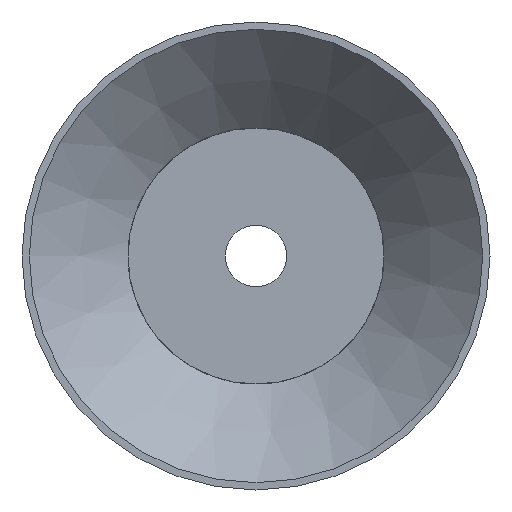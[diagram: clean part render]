
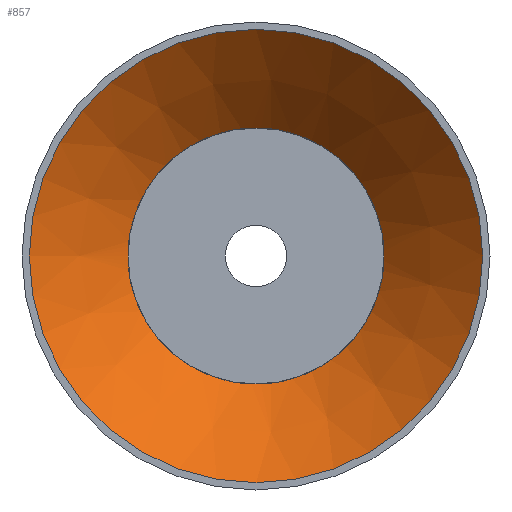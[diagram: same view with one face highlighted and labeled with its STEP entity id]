
A CAD part, front view. The second image highlights one B-rep face of the part: STEP entity #857.
In plain terms, the highlighted conical face has half-angle 44.198 degrees and reference radius 30.725 mm.
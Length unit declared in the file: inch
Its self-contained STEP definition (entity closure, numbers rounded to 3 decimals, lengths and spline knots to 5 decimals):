
#120=(
BOUNDED_CURVE()
B_SPLINE_CURVE(2,(#1166,#1167,#1168),.UNSPECIFIED.,.F.,.F.)
B_SPLINE_CURVE_WITH_KNOTS((3,3),(0.,0.02349),.UNSPECIFIED.)
CURVE()
GEOMETRIC_REPRESENTATION_ITEM()
RATIONAL_B_SPLINE_CURVE((1.,1.,1.))
REPRESENTATION_ITEM('')
);
#121=(
BOUNDED_CURVE()
B_SPLINE_CURVE(2,(#1170,#1171,#1172),.UNSPECIFIED.,.F.,.F.)
B_SPLINE_CURVE_WITH_KNOTS((3,3),(0.83056,0.85405),
 .UNSPECIFIED.)
CURVE()
GEOMETRIC_REPRESENTATION_ITEM()
RATIONAL_B_SPLINE_CURVE((1.,1.,1.))
REPRESENTATION_ITEM('')
);
#122=(
BOUNDED_CURVE()
B_SPLINE_CURVE(2,(#1175,#1176,#1177),.UNSPECIFIED.,.F.,.F.)
B_SPLINE_CURVE_WITH_KNOTS((3,3),(0.,0.02349),.UNSPECIFIED.)
CURVE()
GEOMETRIC_REPRESENTATION_ITEM()
RATIONAL_B_SPLINE_CURVE((1.,1.,1.))
REPRESENTATION_ITEM('')
);
#123=(
BOUNDED_CURVE()
B_SPLINE_CURVE(2,(#1179,#1180,#1181),.UNSPECIFIED.,.F.,.F.)
B_SPLINE_CURVE_WITH_KNOTS((3,3),(0.83035,0.85384),
 .UNSPECIFIED.)
CURVE()
GEOMETRIC_REPRESENTATION_ITEM()
RATIONAL_B_SPLINE_CURVE((1.,1.,1.))
REPRESENTATION_ITEM('')
);
#124=(
BOUNDED_CURVE()
B_SPLINE_CURVE(2,(#1185,#1186,#1187),.UNSPECIFIED.,.F.,.F.)
B_SPLINE_CURVE_WITH_KNOTS((3,3),(0.,0.02349),.UNSPECIFIED.)
CURVE()
GEOMETRIC_REPRESENTATION_ITEM()
RATIONAL_B_SPLINE_CURVE((1.,1.,1.))
REPRESENTATION_ITEM('')
);
#125=(
BOUNDED_CURVE()
B_SPLINE_CURVE(2,(#1191,#1192,#1193),.UNSPECIFIED.,.F.,.F.)
B_SPLINE_CURVE_WITH_KNOTS((3,3),(0.83055,0.85403),
 .UNSPECIFIED.)
CURVE()
GEOMETRIC_REPRESENTATION_ITEM()
RATIONAL_B_SPLINE_CURVE((1.,1.,1.))
REPRESENTATION_ITEM('')
);
#126=(
BOUNDED_CURVE()
B_SPLINE_CURVE(2,(#1196,#1197,#1198),.UNSPECIFIED.,.F.,.F.)
B_SPLINE_CURVE_WITH_KNOTS((3,3),(0.,0.02349),.UNSPECIFIED.)
CURVE()
GEOMETRIC_REPRESENTATION_ITEM()
RATIONAL_B_SPLINE_CURVE((1.,1.,1.))
REPRESENTATION_ITEM('')
);
#127=(
BOUNDED_CURVE()
B_SPLINE_CURVE(2,(#1200,#1201,#1202),.UNSPECIFIED.,.F.,.F.)
B_SPLINE_CURVE_WITH_KNOTS((3,3),(0.83061,0.8541),
 .UNSPECIFIED.)
CURVE()
GEOMETRIC_REPRESENTATION_ITEM()
RATIONAL_B_SPLINE_CURVE((1.,1.,1.))
REPRESENTATION_ITEM('')
);
#132=FACE_OUTER_BOUND('',#172,.T.);
#172=EDGE_LOOP('',(#567,#568,#569,#570,#571,#572,#573,#574,#575,#576,#577,
#578,#579,#580,#581,#582,#583,#584,#585,#586,#587));
#212=CIRCLE('',#910,0.86928);
#214=CIRCLE('',#913,0.86928);
#215=CIRCLE('',#915,0.86928);
#217=CIRCLE('',#918,1.55);
#218=CIRCLE('',#919,0.875);
#219=CIRCLE('',#920,0.875);
#220=CIRCLE('',#921,0.875);
#221=CIRCLE('',#922,0.86928);
#222=CIRCLE('',#923,0.875);
#223=CIRCLE('',#924,0.875);
#224=CIRCLE('',#925,1.55);
#253=LINE('',#1163,#284);
#284=VECTOR('',#1001,1.20964);
#310=VERTEX_POINT('',#1133);
#312=VERTEX_POINT('',#1137);
#314=VERTEX_POINT('',#1142);
#316=VERTEX_POINT('',#1146);
#317=VERTEX_POINT('',#1150);
#319=VERTEX_POINT('',#1153);
#321=VERTEX_POINT('',#1159);
#322=VERTEX_POINT('',#1160);
#323=VERTEX_POINT('',#1162);
#324=VERTEX_POINT('',#1164);
#325=VERTEX_POINT('',#1169);
#326=VERTEX_POINT('',#1173);
#327=VERTEX_POINT('',#1178);
#328=VERTEX_POINT('',#1182);
#329=VERTEX_POINT('',#1184);
#330=VERTEX_POINT('',#1188);
#331=VERTEX_POINT('',#1190);
#332=VERTEX_POINT('',#1194);
#333=VERTEX_POINT('',#1199);
#412=EDGE_CURVE('',#312,#310,#212,.T.);
#416=EDGE_CURVE('',#316,#314,#214,.T.);
#418=EDGE_CURVE('',#317,#319,#215,.T.);
#421=EDGE_CURVE('',#321,#322,#217,.T.);
#422=EDGE_CURVE('',#322,#323,#253,.T.);
#423=EDGE_CURVE('',#324,#323,#218,.T.);
#424=EDGE_CURVE('',#310,#324,#120,.T.);
#425=EDGE_CURVE('',#325,#312,#121,.T.);
#426=EDGE_CURVE('',#326,#325,#219,.T.);
#427=EDGE_CURVE('',#319,#326,#122,.T.);
#428=EDGE_CURVE('',#327,#317,#123,.T.);
#429=EDGE_CURVE('',#328,#327,#220,.T.);
#430=EDGE_CURVE('',#329,#328,#124,.T.);
#431=EDGE_CURVE('',#330,#329,#221,.T.);
#432=EDGE_CURVE('',#331,#330,#125,.T.);
#433=EDGE_CURVE('',#332,#331,#222,.T.);
#434=EDGE_CURVE('',#314,#332,#126,.T.);
#435=EDGE_CURVE('',#333,#316,#127,.T.);
#436=EDGE_CURVE('',#323,#333,#223,.T.);
#437=EDGE_CURVE('',#322,#321,#224,.T.);
#567=ORIENTED_EDGE('',*,*,#421,.T.);
#568=ORIENTED_EDGE('',*,*,#422,.T.);
#569=ORIENTED_EDGE('',*,*,#423,.F.);
#570=ORIENTED_EDGE('',*,*,#424,.F.);
#571=ORIENTED_EDGE('',*,*,#412,.F.);
#572=ORIENTED_EDGE('',*,*,#425,.F.);
#573=ORIENTED_EDGE('',*,*,#426,.F.);
#574=ORIENTED_EDGE('',*,*,#427,.F.);
#575=ORIENTED_EDGE('',*,*,#418,.F.);
#576=ORIENTED_EDGE('',*,*,#428,.F.);
#577=ORIENTED_EDGE('',*,*,#429,.F.);
#578=ORIENTED_EDGE('',*,*,#430,.F.);
#579=ORIENTED_EDGE('',*,*,#431,.F.);
#580=ORIENTED_EDGE('',*,*,#432,.F.);
#581=ORIENTED_EDGE('',*,*,#433,.F.);
#582=ORIENTED_EDGE('',*,*,#434,.F.);
#583=ORIENTED_EDGE('',*,*,#416,.F.);
#584=ORIENTED_EDGE('',*,*,#435,.F.);
#585=ORIENTED_EDGE('',*,*,#436,.F.);
#586=ORIENTED_EDGE('',*,*,#422,.F.);
#587=ORIENTED_EDGE('',*,*,#437,.T.);
#850=CONICAL_SURFACE('',#917,1.20964,0.771);
#857=ADVANCED_FACE('',(#132),#850,.F.);
#910=AXIS2_PLACEMENT_3D('',#1139,#979,#980);
#913=AXIS2_PLACEMENT_3D('',#1148,#987,#988);
#915=AXIS2_PLACEMENT_3D('',#1154,#992,#993);
#917=AXIS2_PLACEMENT_3D('',#1158,#997,#998);
#918=AXIS2_PLACEMENT_3D('',#1161,#999,#1000);
#919=AXIS2_PLACEMENT_3D('',#1165,#1002,#1003);
#920=AXIS2_PLACEMENT_3D('',#1174,#1004,#1005);
#921=AXIS2_PLACEMENT_3D('',#1183,#1006,#1007);
#922=AXIS2_PLACEMENT_3D('',#1189,#1008,#1009);
#923=AXIS2_PLACEMENT_3D('',#1195,#1010,#1011);
#924=AXIS2_PLACEMENT_3D('',#1203,#1012,#1013);
#925=AXIS2_PLACEMENT_3D('',#1204,#1014,#1015);
#979=DIRECTION('center_axis',(0.,-1.,0.));
#980=DIRECTION('ref_axis',(1.,0.,0.));
#987=DIRECTION('center_axis',(0.,-1.,0.));
#988=DIRECTION('ref_axis',(1.,0.,0.));
#992=DIRECTION('center_axis',(0.,-1.,0.));
#993=DIRECTION('ref_axis',(1.,0.,0.));
#997=DIRECTION('center_axis',(0.,-1.,0.));
#998=DIRECTION('ref_axis',(1.,0.,0.));
#999=DIRECTION('center_axis',(0.,-1.,0.));
#1000=DIRECTION('ref_axis',(1.,0.,0.));
#1001=DIRECTION('',(0.697,0.717,0.));
#1002=DIRECTION('center_axis',(0.,-1.,0.));
#1003=DIRECTION('ref_axis',(1.,0.,0.));
#1004=DIRECTION('center_axis',(0.,-1.,0.));
#1005=DIRECTION('ref_axis',(1.,0.,0.));
#1006=DIRECTION('center_axis',(0.,-1.,0.));
#1007=DIRECTION('ref_axis',(1.,0.,0.));
#1008=DIRECTION('center_axis',(0.,-1.,0.));
#1009=DIRECTION('ref_axis',(1.,0.,0.));
#1010=DIRECTION('center_axis',(0.,-1.,0.));
#1011=DIRECTION('ref_axis',(1.,0.,0.));
#1012=DIRECTION('center_axis',(0.,-1.,0.));
#1013=DIRECTION('ref_axis',(1.,0.,0.));
#1014=DIRECTION('center_axis',(0.,-1.,0.));
#1015=DIRECTION('ref_axis',(1.,0.,0.));
#1133=CARTESIAN_POINT('',(-0.86351,0.7,0.10001));
#1137=CARTESIAN_POINT('',(-0.10002,0.7,0.86351));
#1139=CARTESIAN_POINT('Origin',(0.,0.7,0.));
#1142=CARTESIAN_POINT('',(-0.09998,0.7,-0.86351));
#1146=CARTESIAN_POINT('',(-0.86352,0.7,-0.09988));
#1148=CARTESIAN_POINT('Origin',(0.,0.7,0.));
#1150=CARTESIAN_POINT('',(0.86349,0.7,0.1002));
#1153=CARTESIAN_POINT('',(0.10007,0.7,0.8635));
#1154=CARTESIAN_POINT('Origin',(0.,0.7,0.));
#1158=CARTESIAN_POINT('Origin',(0.,0.34998,0.));
#1159=CARTESIAN_POINT('',(1.55,-0.00004,0.));
#1160=CARTESIAN_POINT('',(-1.55,-0.00004,0.));
#1161=CARTESIAN_POINT('Origin',(0.,-0.00004,0.));
#1162=CARTESIAN_POINT('',(-0.875,0.69412,0.));
#1163=CARTESIAN_POINT('',(-1.20964,0.34998,0.));
#1164=CARTESIAN_POINT('',(-0.86927,0.69412,0.10001));
#1165=CARTESIAN_POINT('Origin',(0.,0.69412,0.));
#1166=CARTESIAN_POINT('Ctrl Pts',(-0.86351,0.7,0.10001));
#1167=CARTESIAN_POINT('Ctrl Pts',(-0.86638,0.69707,
0.10001));
#1168=CARTESIAN_POINT('Ctrl Pts',(-0.86927,0.69412,
0.10001));
#1169=CARTESIAN_POINT('',(-0.10002,0.69412,0.86926));
#1170=CARTESIAN_POINT('Ctrl Pts',(-0.10002,0.69412,
0.86926));
#1171=CARTESIAN_POINT('Ctrl Pts',(-0.10002,0.69707,
0.86638));
#1172=CARTESIAN_POINT('Ctrl Pts',(-0.10002,0.7,0.86351));
#1173=CARTESIAN_POINT('',(0.10007,0.69412,0.86926));
#1174=CARTESIAN_POINT('Origin',(0.,0.69412,0.));
#1175=CARTESIAN_POINT('Ctrl Pts',(0.10007,0.7,0.8635));
#1176=CARTESIAN_POINT('Ctrl Pts',(0.10007,0.69707,0.86637));
#1177=CARTESIAN_POINT('Ctrl Pts',(0.10007,0.69412,0.86926));
#1178=CARTESIAN_POINT('',(0.86924,0.69412,0.1002));
#1179=CARTESIAN_POINT('Ctrl Pts',(0.86924,0.69412,0.1002));
#1180=CARTESIAN_POINT('Ctrl Pts',(0.86636,0.69707,0.1002));
#1181=CARTESIAN_POINT('Ctrl Pts',(0.86349,0.7,0.1002));
#1182=CARTESIAN_POINT('',(0.86928,0.69412,-0.09987));
#1183=CARTESIAN_POINT('Origin',(0.,0.69412,0.));
#1184=CARTESIAN_POINT('',(0.86352,0.7,-0.09988));
#1185=CARTESIAN_POINT('Ctrl Pts',(0.86352,0.7,-0.09988));
#1186=CARTESIAN_POINT('Ctrl Pts',(0.86639,0.69707,-0.09988));
#1187=CARTESIAN_POINT('Ctrl Pts',(0.86928,0.69412,-0.09987));
#1188=CARTESIAN_POINT('',(0.09993,0.7,-0.86352));
#1189=CARTESIAN_POINT('Origin',(0.,0.7,0.));
#1190=CARTESIAN_POINT('',(0.09993,0.69412,-0.86928));
#1191=CARTESIAN_POINT('Ctrl Pts',(0.09993,0.69412,
-0.86928));
#1192=CARTESIAN_POINT('Ctrl Pts',(0.09993,0.69707,-0.86639));
#1193=CARTESIAN_POINT('Ctrl Pts',(0.09993,0.7,
-0.86352));
#1194=CARTESIAN_POINT('',(-0.09998,0.69412,-0.86927));
#1195=CARTESIAN_POINT('Origin',(0.,0.69412,0.));
#1196=CARTESIAN_POINT('Ctrl Pts',(-0.09998,0.7,
-0.86351));
#1197=CARTESIAN_POINT('Ctrl Pts',(-0.09998,0.69707,
-0.86638));
#1198=CARTESIAN_POINT('Ctrl Pts',(-0.09998,0.69412,
-0.86927));
#1199=CARTESIAN_POINT('',(-0.86928,0.69412,-0.09988));
#1200=CARTESIAN_POINT('Ctrl Pts',(-0.86928,0.69412,
-0.09988));
#1201=CARTESIAN_POINT('Ctrl Pts',(-0.86639,0.69707,
-0.09988));
#1202=CARTESIAN_POINT('Ctrl Pts',(-0.86352,0.7,
-0.09988));
#1203=CARTESIAN_POINT('Origin',(0.,0.69412,0.));
#1204=CARTESIAN_POINT('Origin',(0.,-0.00004,0.));
